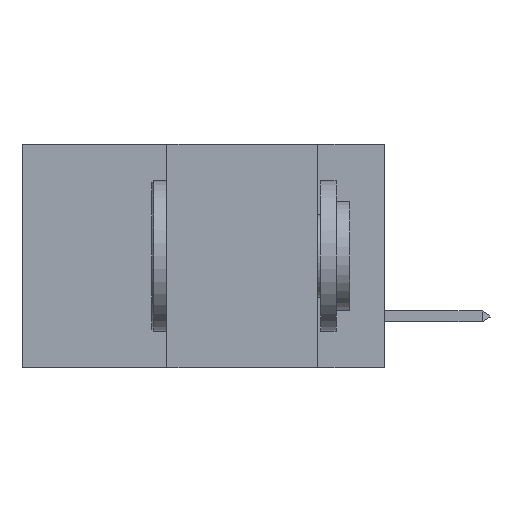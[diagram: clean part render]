
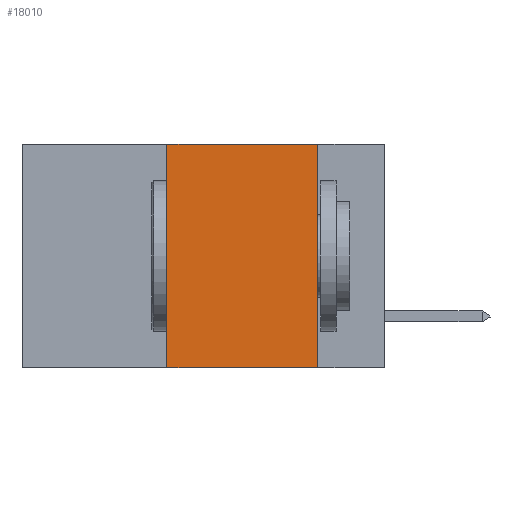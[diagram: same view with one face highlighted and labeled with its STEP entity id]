
A CAD part, left-side view. The second image highlights one B-rep face of the part: STEP entity #18010.
In plain terms, the highlighted planar face has unit normal (-1, 0, 0).
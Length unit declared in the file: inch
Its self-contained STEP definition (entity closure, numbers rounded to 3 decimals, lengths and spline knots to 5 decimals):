
#162 = LINE ( 'NONE', #10608, #13193 ) ;
#632 = AXIS2_PLACEMENT_3D ( 'NONE', #13225, #4794, #4911 ) ;
#1125 = EDGE_CURVE ( 'NONE', #5385, #17244, #8822, .T. ) ;
#2000 = CARTESIAN_POINT ( 'NONE',  ( 0., 0.6, -0.37 ) ) ;
#2613 = ORIENTED_EDGE ( 'NONE', *, *, #14233, .T. ) ;
#2756 = ORIENTED_EDGE ( 'NONE', *, *, #3293, .F. ) ;
#3293 = EDGE_CURVE ( 'NONE', #13846, #13712, #162, .T. ) ;
#3928 = DIRECTION ( 'NONE',  ( 0., 0., -1. ) ) ;
#4656 = VECTOR ( 'NONE', #9396, 39.37008 ) ;
#4794 = DIRECTION ( 'NONE',  ( 1., 0., 0. ) ) ;
#4911 = DIRECTION ( 'NONE',  ( 0., 0., -1. ) ) ;
#5385 = VERTEX_POINT ( 'NONE', #12331 ) ;
#6198 = DIRECTION ( 'NONE',  ( 0., -1., 0. ) ) ;
#6860 = VECTOR ( 'NONE', #6198, 39.37008 ) ;
#7147 = CARTESIAN_POINT ( 'NONE',  ( 0., 0.36, 0. ) ) ;
#7730 = ORIENTED_EDGE ( 'NONE', *, *, #1125, .F. ) ;
#8093 = ORIENTED_EDGE ( 'NONE', *, *, #16692, .F. ) ;
#8822 = LINE ( 'NONE', #12253, #4656 ) ;
#9396 = DIRECTION ( 'NONE',  ( 0., 0., 1. ) ) ;
#10036 = CARTESIAN_POINT ( 'NONE',  ( 0., 0.11, -0.37 ) ) ;
#10608 = CARTESIAN_POINT ( 'NONE',  ( 0., 0.11, 0. ) ) ;
#10839 = DIRECTION ( 'NONE',  ( 0., -1., 0. ) ) ;
#11727 = FACE_OUTER_BOUND ( 'NONE', #15511, .T. ) ;
#12253 = CARTESIAN_POINT ( 'NONE',  ( 0., 0.36, 0. ) ) ;
#12331 = CARTESIAN_POINT ( 'NONE',  ( 0., 0.36, -0.37 ) ) ;
#13193 = VECTOR ( 'NONE', #3928, 39.37008 ) ;
#13225 = CARTESIAN_POINT ( 'NONE',  ( 0., 0.6, 0. ) ) ;
#13712 = VERTEX_POINT ( 'NONE', #10036 ) ;
#13846 = VERTEX_POINT ( 'NONE', #15817 ) ;
#14233 = EDGE_CURVE ( 'NONE', #5385, #13712, #17913, .T. ) ;
#14859 = PLANE ( 'NONE',  #632 ) ;
#14951 = CARTESIAN_POINT ( 'NONE',  ( 0., 0.6, 0. ) ) ;
#15511 = EDGE_LOOP ( 'NONE', ( #2756, #8093, #7730, #2613 ) ) ;
#15817 = CARTESIAN_POINT ( 'NONE',  ( 0., 0.11, 0. ) ) ;
#16692 = EDGE_CURVE ( 'NONE', #17244, #13846, #17588, .T. ) ;
#16928 = VECTOR ( 'NONE', #10839, 39.37008 ) ;
#17244 = VERTEX_POINT ( 'NONE', #7147 ) ;
#17588 = LINE ( 'NONE', #14951, #16928 ) ;
#17913 = LINE ( 'NONE', #2000, #6860 ) ;
#18010 = ADVANCED_FACE ( 'NONE', ( #11727 ), #14859, .F. ) ;
